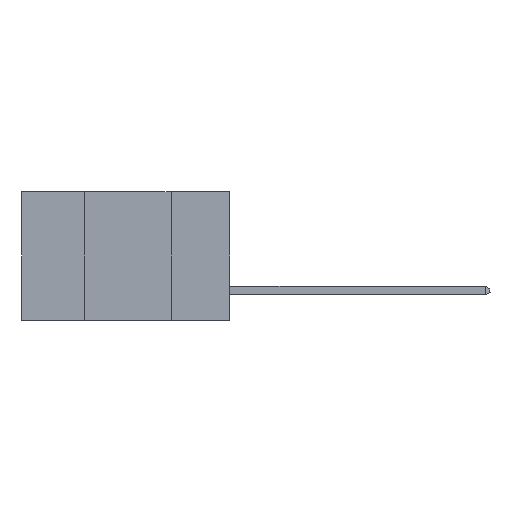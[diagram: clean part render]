
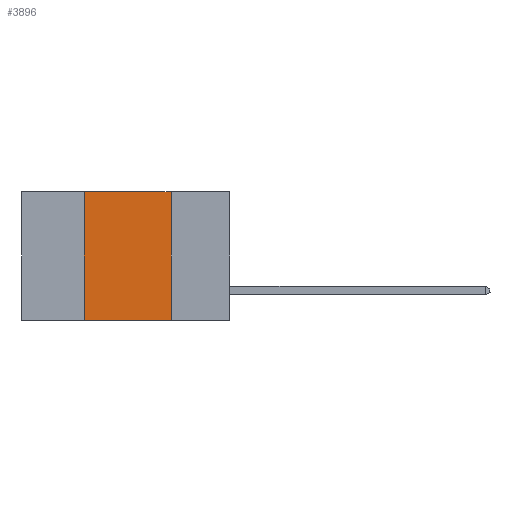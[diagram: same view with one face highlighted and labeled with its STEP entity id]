
A CAD part, left-side view. The second image highlights one B-rep face of the part: STEP entity #3896.
In plain terms, the highlighted planar face has unit normal (-1, 0, 0).
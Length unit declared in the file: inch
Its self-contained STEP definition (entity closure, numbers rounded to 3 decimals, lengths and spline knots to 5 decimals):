
#563 = CARTESIAN_POINT ( 'NONE',  ( 0., 0.17, 0. ) ) ;
#1224 = EDGE_CURVE ( 'NONE', #19954, #18456, #5642, .T. ) ;
#1276 = CARTESIAN_POINT ( 'NONE',  ( 0., 0.42, 0. ) ) ;
#1279 = VECTOR ( 'NONE', #15586, 39.37008 ) ;
#1410 = CARTESIAN_POINT ( 'NONE',  ( 0., 0.6, 0. ) ) ;
#1742 = VECTOR ( 'NONE', #10125, 39.37008 ) ;
#2443 = VERTEX_POINT ( 'NONE', #563 ) ;
#3097 = FACE_OUTER_BOUND ( 'NONE', #19381, .T. ) ;
#3266 = CARTESIAN_POINT ( 'NONE',  ( 0., 0.6, -0.37 ) ) ;
#3896 = ADVANCED_FACE ( 'NONE', ( #3097 ), #11709, .F. ) ;
#5111 = DIRECTION ( 'NONE',  ( 0., 0., -1. ) ) ;
#5642 = LINE ( 'NONE', #16849, #16552 ) ;
#5662 = AXIS2_PLACEMENT_3D ( 'NONE', #1410, #16906, #5111 ) ;
#6702 = CARTESIAN_POINT ( 'NONE',  ( 0., 0.17, 0. ) ) ;
#6765 = CARTESIAN_POINT ( 'NONE',  ( 0., 0.42, -0.37 ) ) ;
#6843 = VECTOR ( 'NONE', #16777, 39.37008 ) ;
#9812 = ORIENTED_EDGE ( 'NONE', *, *, #14146, .F. ) ;
#10125 = DIRECTION ( 'NONE',  ( 0., 0., -1. ) ) ;
#10838 = LINE ( 'NONE', #3266, #6843 ) ;
#11709 = PLANE ( 'NONE',  #5662 ) ;
#12014 = DIRECTION ( 'NONE',  ( 0., 0., 1. ) ) ;
#12865 = EDGE_CURVE ( 'NONE', #18456, #2443, #19826, .T. ) ;
#13553 = ORIENTED_EDGE ( 'NONE', *, *, #14466, .T. ) ;
#14146 = EDGE_CURVE ( 'NONE', #2443, #19416, #14768, .T. ) ;
#14466 = EDGE_CURVE ( 'NONE', #19954, #19416, #10838, .T. ) ;
#14768 = LINE ( 'NONE', #6702, #1742 ) ;
#15586 = DIRECTION ( 'NONE',  ( 0., -1., 0. ) ) ;
#15627 = ORIENTED_EDGE ( 'NONE', *, *, #1224, .F. ) ;
#16552 = VECTOR ( 'NONE', #12014, 39.37008 ) ;
#16777 = DIRECTION ( 'NONE',  ( 0., -1., 0. ) ) ;
#16849 = CARTESIAN_POINT ( 'NONE',  ( 0., 0.42, 0. ) ) ;
#16906 = DIRECTION ( 'NONE',  ( 1., 0., 0. ) ) ;
#18456 = VERTEX_POINT ( 'NONE', #1276 ) ;
#18646 = CARTESIAN_POINT ( 'NONE',  ( 0., 0.6, 0. ) ) ;
#19034 = CARTESIAN_POINT ( 'NONE',  ( 0., 0.17, -0.37 ) ) ;
#19381 = EDGE_LOOP ( 'NONE', ( #9812, #21687, #15627, #13553 ) ) ;
#19416 = VERTEX_POINT ( 'NONE', #19034 ) ;
#19826 = LINE ( 'NONE', #18646, #1279 ) ;
#19954 = VERTEX_POINT ( 'NONE', #6765 ) ;
#21687 = ORIENTED_EDGE ( 'NONE', *, *, #12865, .F. ) ;
